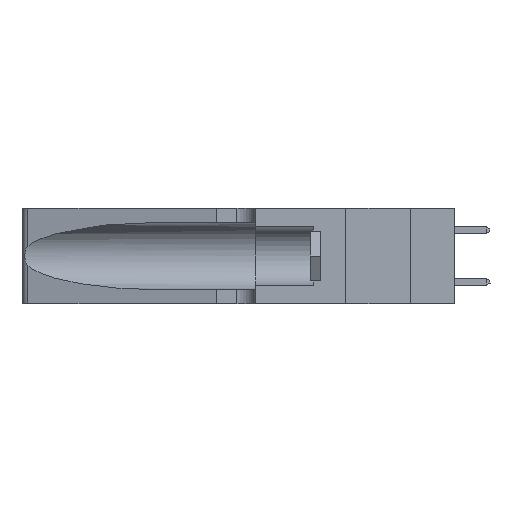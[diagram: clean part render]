
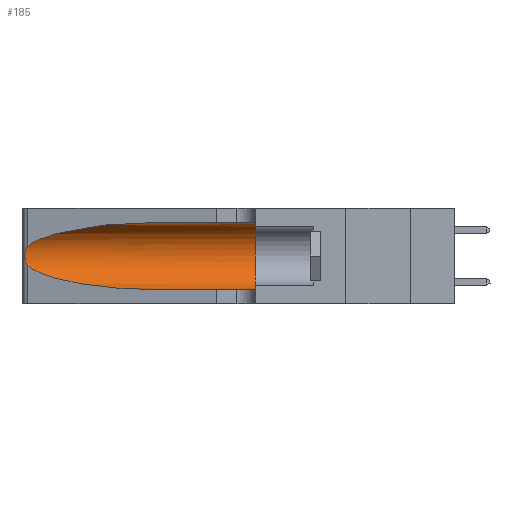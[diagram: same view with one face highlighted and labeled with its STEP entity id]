
A CAD part, left-side view. The second image highlights one B-rep face of the part: STEP entity #185.
In plain terms, the highlighted cylindrical face has radius 3.308 mm (diameter 6.617 mm), a partial arc.
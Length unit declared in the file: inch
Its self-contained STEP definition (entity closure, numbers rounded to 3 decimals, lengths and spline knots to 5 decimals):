
#185 = ADVANCED_FACE ( 'NONE', ( #17837 ), #20704, .F. ) ;
#277 = ORIENTED_EDGE ( 'NONE', *, *, #8537, .T. ) ;
#391 =( BOUNDED_CURVE ( )  B_SPLINE_CURVE ( 3, ( #3434, #834, #13689, #17364 ),
 .UNSPECIFIED., .F., .T. ) 
 B_SPLINE_CURVE_WITH_KNOTS ( ( 4, 4 ),
 ( 1.5708, 2.84003 ),
 .UNSPECIFIED. ) 
 CURVE ( )  GEOMETRIC_REPRESENTATION_ITEM ( )  RATIONAL_B_SPLINE_CURVE ( ( 1., 0.87, 0.87, 1. ) ) 
 REPRESENTATION_ITEM ( '' )  );
#476 = ORIENTED_EDGE ( 'NONE', *, *, #16454, .T. ) ;
#832 = CARTESIAN_POINT ( 'NONE',  ( 0.1305, 0.35, 0.31525 ) ) ;
#834 = CARTESIAN_POINT ( 'NONE',  ( 0.18966, 0.96281, 0.31525 ) ) ;
#1319 = DIRECTION ( 'NONE',  ( 0., -1., 0. ) ) ;
#1518 = VERTEX_POINT ( 'NONE', #11686 ) ;
#2322 = DIRECTION ( 'NONE',  ( 0., 1., 0. ) ) ;
#2536 = AXIS2_PLACEMENT_3D ( 'NONE', #7724, #10314, #31305 ) ;
#2552 = CARTESIAN_POINT ( 'NONE',  ( 0.25639, 1.23186, 0.15144 ) ) ;
#3434 = CARTESIAN_POINT ( 'NONE',  ( 0.1305, 0.72297, 0.31525 ) ) ;
#4687 = EDGE_LOOP ( 'NONE', ( #277, #26394, #5096, #476, #16178, #27379 ) ) ;
#5096 = ORIENTED_EDGE ( 'NONE', *, *, #11469, .T. ) ;
#7030 = CARTESIAN_POINT ( 'NONE',  ( 0.25787, 1.23484, 0.2124 ) ) ;
#7167 = CARTESIAN_POINT ( 'NONE',  ( 0.26018, 1.23835, 0.19895 ) ) ;
#7555 = CARTESIAN_POINT ( 'NONE',  ( 0.25487, 1.22718, 0.14631 ) ) ;
#7724 = CARTESIAN_POINT ( 'NONE',  ( 0.1305, 1.61858, 0.185 ) ) ;
#8082 = CARTESIAN_POINT ( 'NONE',  ( 0.26017, 1.23833, 0.17102 ) ) ;
#8537 = EDGE_CURVE ( 'NONE', #23749, #12141, #391, .T. ) ;
#9053 =( BOUNDED_CURVE ( )  B_SPLINE_CURVE ( 3, ( #17848, #30974, #33526, #17732 ),
 .UNSPECIFIED., .F., .F. ) 
 B_SPLINE_CURVE_WITH_KNOTS ( ( 4, 4 ),
 ( 3.44316, 4.71239 ),
 .UNSPECIFIED. ) 
 CURVE ( )  GEOMETRIC_REPRESENTATION_ITEM ( )  RATIONAL_B_SPLINE_CURVE ( ( 1., 0.87, 0.87, 1. ) ) 
 REPRESENTATION_ITEM ( '' )  );
#9196 = CARTESIAN_POINT ( 'NONE',  ( 0.25555, 1.22994, 0.2215 ) ) ;
#9241 = DIRECTION ( 'NONE',  ( 0., -1., 0. ) ) ;
#10019 = CARTESIAN_POINT ( 'NONE',  ( 0.25639, 1.23184, 0.21858 ) ) ;
#10314 = DIRECTION ( 'NONE',  ( 0., -1., 0. ) ) ;
#11312 = VECTOR ( 'NONE', #9241, 39.37008 ) ;
#11469 = EDGE_CURVE ( 'NONE', #20646, #20420, #9053, .T. ) ;
#11686 = CARTESIAN_POINT ( 'NONE',  ( 0.1305, 0.35, 0.05475 ) ) ;
#12141 = VERTEX_POINT ( 'NONE', #32971 ) ;
#12428 = CARTESIAN_POINT ( 'NONE',  ( 0.26075, 1.23896, 0.19203 ) ) ;
#12668 = CARTESIAN_POINT ( 'NONE',  ( 0.25854, 1.2359, 0.20912 ) ) ;
#13689 = CARTESIAN_POINT ( 'NONE',  ( 0.2373, 1.15595, 0.28018 ) ) ;
#14988 = CARTESIAN_POINT ( 'NONE',  ( 0.1305, 1.61858, 0.05475 ) ) ;
#15311 = CARTESIAN_POINT ( 'NONE',  ( 0.1305, 0.35, 0.185 ) ) ;
#16178 = ORIENTED_EDGE ( 'NONE', *, *, #31101, .F. ) ;
#16454 = EDGE_CURVE ( 'NONE', #20420, #1518, #27216, .T. ) ;
#17364 = CARTESIAN_POINT ( 'NONE',  ( 0.25487, 1.22718, 0.22369 ) ) ;
#17732 = CARTESIAN_POINT ( 'NONE',  ( 0.1305, 0.72297, 0.05475 ) ) ;
#17837 = FACE_OUTER_BOUND ( 'NONE', #4687, .T. ) ;
#17848 = CARTESIAN_POINT ( 'NONE',  ( 0.25487, 1.22718, 0.14631 ) ) ;
#18088 = CARTESIAN_POINT ( 'NONE',  ( 0.25789, 1.23486, 0.15765 ) ) ;
#18831 = VERTEX_POINT ( 'NONE', #832 ) ;
#19830 = CARTESIAN_POINT ( 'NONE',  ( 0.1305, 1.61858, 0.31525 ) ) ;
#20305 = EDGE_CURVE ( 'NONE', #12141, #20646, #33027, .T. ) ;
#20371 = VECTOR ( 'NONE', #1319, 39.37008 ) ;
#20420 = VERTEX_POINT ( 'NONE', #24546 ) ;
#20646 = VERTEX_POINT ( 'NONE', #7555 ) ;
#20704 = CYLINDRICAL_SURFACE ( 'NONE', #2536, 0.13025 ) ;
#20943 = DIRECTION ( 'NONE',  ( 0., 0., 1. ) ) ;
#21787 = AXIS2_PLACEMENT_3D ( 'NONE', #15311, #2322, #20943 ) ;
#23749 = VERTEX_POINT ( 'NONE', #29410 ) ;
#24546 = CARTESIAN_POINT ( 'NONE',  ( 0.1305, 0.72297, 0.05475 ) ) ;
#26394 = ORIENTED_EDGE ( 'NONE', *, *, #20305, .T. ) ;
#26603 = CARTESIAN_POINT ( 'NONE',  ( 0.25487, 1.22718, 0.14631 ) ) ;
#27216 = LINE ( 'NONE', #14988, #20371 ) ;
#27379 = ORIENTED_EDGE ( 'NONE', *, *, #27676, .F. ) ;
#27617 = CARTESIAN_POINT ( 'NONE',  ( 0.25487, 1.22718, 0.22369 ) ) ;
#27676 = EDGE_CURVE ( 'NONE', #23749, #18831, #31112, .T. ) ;
#29410 = CARTESIAN_POINT ( 'NONE',  ( 0.1305, 0.72297, 0.31525 ) ) ;
#30974 = CARTESIAN_POINT ( 'NONE',  ( 0.2373, 1.15595, 0.08982 ) ) ;
#31101 = EDGE_CURVE ( 'NONE', #18831, #1518, #32107, .T. ) ;
#31112 = LINE ( 'NONE', #19830, #11312 ) ;
#31305 = DIRECTION ( 'NONE',  ( 0., 0., -1. ) ) ;
#31564 = CARTESIAN_POINT ( 'NONE',  ( 0.26075, 1.23896, 0.178 ) ) ;
#32107 = CIRCLE ( 'NONE', #21787, 0.13025 ) ;
#32971 = CARTESIAN_POINT ( 'NONE',  ( 0.25487, 1.22718, 0.22369 ) ) ;
#33027 = B_SPLINE_CURVE_WITH_KNOTS ( 'NONE', 3,
 ( #27617, #9196, #10019, #7030, #12668, #7167, #12428, #31564, #8082, #33984, #18088, #2552, #33882, #26603 ),
 .UNSPECIFIED., .F., .F.,
 ( 4, 2, 2, 2, 2, 2, 4 ),
 ( 0., 0.00027, 0.00053, 0.00107, 0.0016, 0.00187, 0.00214 ),
 .UNSPECIFIED. ) ;
#33526 = CARTESIAN_POINT ( 'NONE',  ( 0.18966, 0.96281, 0.05475 ) ) ;
#33882 = CARTESIAN_POINT ( 'NONE',  ( 0.25555, 1.22993, 0.14849 ) ) ;
#33984 = CARTESIAN_POINT ( 'NONE',  ( 0.25856, 1.23593, 0.16098 ) ) ;
